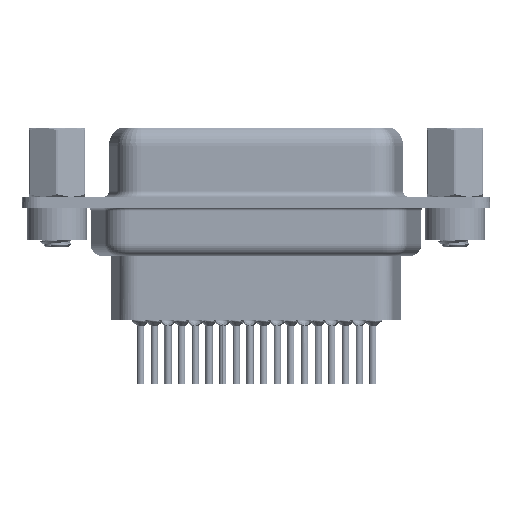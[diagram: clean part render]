
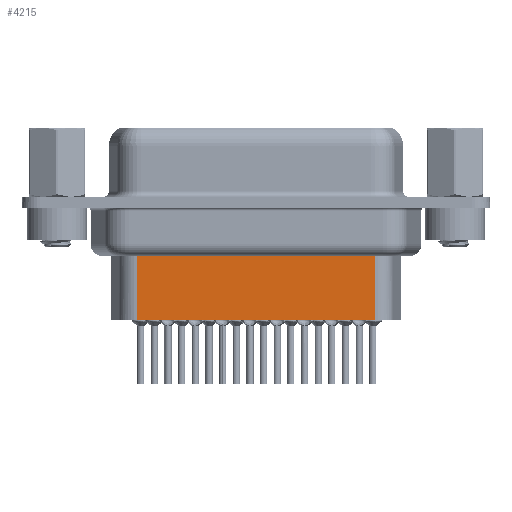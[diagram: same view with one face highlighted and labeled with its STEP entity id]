
A CAD part, front view. The second image highlights one B-rep face of the part: STEP entity #4215.
In plain terms, the highlighted planar face has unit normal (0, -1, 0).
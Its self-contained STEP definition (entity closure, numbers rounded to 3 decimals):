
#81 = CARTESIAN_POINT ( 'NONE',  ( 26.629, -3.5, -3.1 ) ) ;
#2049 = EDGE_CURVE ( 'NONE', #7488, #11727, #26064, .T. ) ;
#3148 = CARTESIAN_POINT ( 'NONE',  ( 26.629, -3.5, -4.097 ) ) ;
#3788 = ORIENTED_EDGE ( 'NONE', *, *, #2049, .F. ) ;
#3926 = CARTESIAN_POINT ( 'NONE',  ( 6.691, -3.5, -4.097 ) ) ;
#4215 = ADVANCED_FACE ( 'NONE', ( #15477 ), #9051, .T. ) ;
#4718 = DIRECTION ( 'NONE',  ( -1., 0., 0. ) ) ;
#4739 = VECTOR ( 'NONE', #14863, 1000. ) ;
#5342 = EDGE_CURVE ( 'NONE', #11727, #36512, #27654, .T. ) ;
#5682 = EDGE_LOOP ( 'NONE', ( #3788, #11891, #25149, #32308 ) ) ;
#6784 = CARTESIAN_POINT ( 'NONE',  ( 6.444, -3.5, -4.097 ) ) ;
#7488 = VERTEX_POINT ( 'NONE', #3148 ) ;
#9051 = PLANE ( 'NONE',  #21872 ) ;
#11727 = VERTEX_POINT ( 'NONE', #18749 ) ;
#11891 = ORIENTED_EDGE ( 'NONE', *, *, #16237, .T. ) ;
#12021 = LINE ( 'NONE', #21465, #13820 ) ;
#13820 = VECTOR ( 'NONE', #15422, 1000. ) ;
#14863 = DIRECTION ( 'NONE',  ( 0., 0., -1. ) ) ;
#15422 = DIRECTION ( 'NONE',  ( 0., 0., -1. ) ) ;
#15477 = FACE_OUTER_BOUND ( 'NONE', #5682, .T. ) ;
#16237 = EDGE_CURVE ( 'NONE', #7488, #35122, #21162, .T. ) ;
#16280 = CARTESIAN_POINT ( 'NONE',  ( 6.691, -3.5, -9.85 ) ) ;
#17767 = DIRECTION ( 'NONE',  ( 1., 0., 0. ) ) ;
#18319 = DIRECTION ( 'NONE',  ( 0., -1., 0. ) ) ;
#18749 = CARTESIAN_POINT ( 'NONE',  ( 26.629, -3.5, -9.85 ) ) ;
#20618 = DIRECTION ( 'NONE',  ( -1., 0., 0. ) ) ;
#21162 = LINE ( 'NONE', #6784, #22229 ) ;
#21465 = CARTESIAN_POINT ( 'NONE',  ( 6.691, -3.5, -3.1 ) ) ;
#21872 = AXIS2_PLACEMENT_3D ( 'NONE', #29902, #18319, #17767 ) ;
#22229 = VECTOR ( 'NONE', #20618, 1000. ) ;
#22303 = EDGE_CURVE ( 'NONE', #35122, #36512, #12021, .T. ) ;
#25149 = ORIENTED_EDGE ( 'NONE', *, *, #22303, .T. ) ;
#26064 = LINE ( 'NONE', #81, #4739 ) ;
#27654 = LINE ( 'NONE', #16280, #32715 ) ;
#29902 = CARTESIAN_POINT ( 'NONE',  ( 6.691, -3.5, -3.1 ) ) ;
#30023 = CARTESIAN_POINT ( 'NONE',  ( 6.691, -3.5, -9.85 ) ) ;
#32308 = ORIENTED_EDGE ( 'NONE', *, *, #5342, .F. ) ;
#32715 = VECTOR ( 'NONE', #4718, 1000. ) ;
#35122 = VERTEX_POINT ( 'NONE', #3926 ) ;
#36512 = VERTEX_POINT ( 'NONE', #30023 ) ;
